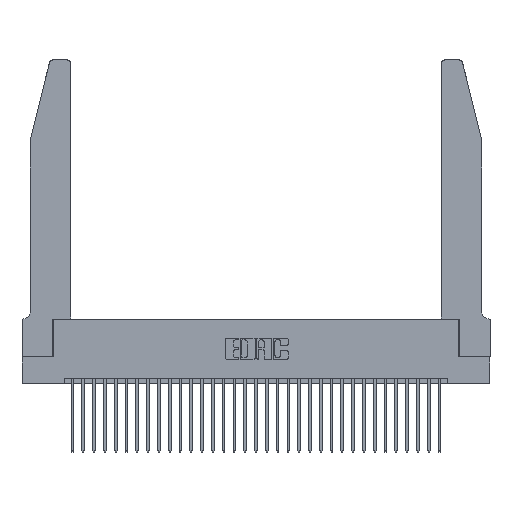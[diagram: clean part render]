
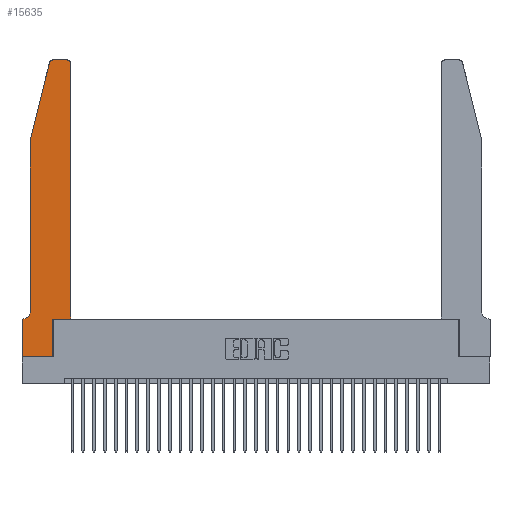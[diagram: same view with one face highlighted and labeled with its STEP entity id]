
A CAD part, top view. The second image highlights one B-rep face of the part: STEP entity #15635.
In plain terms, the highlighted planar face has unit normal (0, 0, 1).
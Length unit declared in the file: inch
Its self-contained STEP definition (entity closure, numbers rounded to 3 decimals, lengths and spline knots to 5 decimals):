
#44 = ORIENTED_EDGE ( 'NONE', *, *, #20738, .T. ) ;
#1139 = EDGE_CURVE ( 'NONE', #29773, #28046, #31477, .T. ) ;
#1188 = DIRECTION ( 'NONE',  ( 1., 0., 0. ) ) ;
#1494 = DIRECTION ( 'NONE',  ( -1., 0., 0. ) ) ;
#2541 = LINE ( 'NONE', #8914, #22232 ) ;
#2862 = ORIENTED_EDGE ( 'NONE', *, *, #24527, .T. ) ;
#3100 = AXIS2_PLACEMENT_3D ( 'NONE', #10917, #31231, #28547 ) ;
#3407 = DIRECTION ( 'NONE',  ( 0., 1., 0. ) ) ;
#3511 = LINE ( 'NONE', #30862, #12816 ) ;
#3593 = ORIENTED_EDGE ( 'NONE', *, *, #30629, .T. ) ;
#3734 = VERTEX_POINT ( 'NONE', #26881 ) ;
#4001 = CARTESIAN_POINT ( 'NONE',  ( 0.2865, 0.35, 0.37 ) ) ;
#4684 = ORIENTED_EDGE ( 'NONE', *, *, #8996, .T. ) ;
#5107 = DIRECTION ( 'NONE',  ( 0., 0., -1. ) ) ;
#5984 = EDGE_CURVE ( 'NONE', #23212, #20855, #3511, .T. ) ;
#6069 = VERTEX_POINT ( 'NONE', #24100 ) ;
#6138 = CARTESIAN_POINT ( 'NONE',  ( 0.284, 2.75, 0.37 ) ) ;
#7278 = CARTESIAN_POINT ( 'NONE',  ( 0.0055, 0.42, 0.37 ) ) ;
#7565 = ORIENTED_EDGE ( 'NONE', *, *, #8165, .T. ) ;
#7807 = LINE ( 'NONE', #10770, #21006 ) ;
#7974 = ORIENTED_EDGE ( 'NONE', *, *, #15276, .T. ) ;
#7991 = EDGE_LOOP ( 'NONE', ( #7565, #32220, #29162, #4684, #2862, #28185, #7974, #3593, #24449, #31162, #17124, #44 ) ) ;
#8165 = EDGE_CURVE ( 'NONE', #8243, #15471, #18861, .T. ) ;
#8214 = VECTOR ( 'NONE', #21983, 39.37008 ) ;
#8243 = VERTEX_POINT ( 'NONE', #17296 ) ;
#8914 = CARTESIAN_POINT ( 'NONE',  ( 0.4505, 0.35, 0.37 ) ) ;
#8996 = EDGE_CURVE ( 'NONE', #20855, #14563, #14659, .T. ) ;
#9377 = VECTOR ( 'NONE', #3407, 39.37008 ) ;
#10770 = CARTESIAN_POINT ( 'NONE',  ( 0., 0., 0.37 ) ) ;
#10917 = CARTESIAN_POINT ( 'NONE',  ( 0.4205, 2.72, 0.37 ) ) ;
#11290 = DIRECTION ( 'NONE',  ( 1., 0., 0. ) ) ;
#11753 = VERTEX_POINT ( 'NONE', #12841 ) ;
#12213 = EDGE_CURVE ( 'NONE', #29085, #6069, #20867, .T. ) ;
#12527 = VECTOR ( 'NONE', #17691, 39.37008 ) ;
#12816 = VECTOR ( 'NONE', #25686, 39.37008 ) ;
#12841 = CARTESIAN_POINT ( 'NONE',  ( 0., 0., 0.37 ) ) ;
#13200 = CARTESIAN_POINT ( 'NONE',  ( 0.4505, 2.72, 0.37 ) ) ;
#13548 = DIRECTION ( 'NONE',  ( 0., 0., 1. ) ) ;
#13605 = AXIS2_PLACEMENT_3D ( 'NONE', #7278, #5107, #15448 ) ;
#13682 = DIRECTION ( 'NONE',  ( -1., 0., 0. ) ) ;
#13918 = CIRCLE ( 'NONE', #13605, 0.07 ) ;
#14563 = VERTEX_POINT ( 'NONE', #17896 ) ;
#14659 = LINE ( 'NONE', #27059, #26262 ) ;
#15276 = EDGE_CURVE ( 'NONE', #6069, #11753, #7807, .T. ) ;
#15448 = DIRECTION ( 'NONE',  ( -1., 0., 0. ) ) ;
#15471 = VERTEX_POINT ( 'NONE', #6138 ) ;
#15635 = ADVANCED_FACE ( 'NONE', ( #29424 ), #26188, .T. ) ;
#15729 = EDGE_CURVE ( 'NONE', #28046, #3734, #2541, .T. ) ;
#16372 = CARTESIAN_POINT ( 'NONE',  ( 0.0755, 0.35, 0.37 ) ) ;
#16467 = VECTOR ( 'NONE', #1494, 39.37008 ) ;
#16550 = CARTESIAN_POINT ( 'NONE',  ( 0.0055, 0.35, 0.37 ) ) ;
#16721 = AXIS2_PLACEMENT_3D ( 'NONE', #33086, #18148, #20621 ) ;
#16952 = CARTESIAN_POINT ( 'NONE',  ( 0.2865, 0., 0.37 ) ) ;
#17124 = ORIENTED_EDGE ( 'NONE', *, *, #25946, .T. ) ;
#17213 = CARTESIAN_POINT ( 'NONE',  ( 0.0755, 2., 0.37 ) ) ;
#17296 = CARTESIAN_POINT ( 'NONE',  ( 0.4205, 2.75, 0.37 ) ) ;
#17691 = DIRECTION ( 'NONE',  ( 1., 0., 0. ) ) ;
#17896 = CARTESIAN_POINT ( 'NONE',  ( 0.0755, 0.42, 0.37 ) ) ;
#18148 = DIRECTION ( 'NONE',  ( 0., 0., 1. ) ) ;
#18810 = CARTESIAN_POINT ( 'NONE',  ( 0.4505, 0.35, 0.37 ) ) ;
#18861 = LINE ( 'NONE', #24466, #16467 ) ;
#19808 = CIRCLE ( 'NONE', #16721, 0.03 ) ;
#20621 = DIRECTION ( 'NONE',  ( 1., 0., 0. ) ) ;
#20738 = EDGE_CURVE ( 'NONE', #22619, #8243, #25141, .T. ) ;
#20855 = VERTEX_POINT ( 'NONE', #17213 ) ;
#20867 = LINE ( 'NONE', #16372, #26501 ) ;
#21006 = VECTOR ( 'NONE', #28832, 39.37008 ) ;
#21983 = DIRECTION ( 'NONE',  ( 0., 1., 0. ) ) ;
#22232 = VECTOR ( 'NONE', #1188, 39.37008 ) ;
#22619 = VERTEX_POINT ( 'NONE', #13200 ) ;
#23212 = VERTEX_POINT ( 'NONE', #26747 ) ;
#24100 = CARTESIAN_POINT ( 'NONE',  ( 0., 0.35, 0.37 ) ) ;
#24163 = LINE ( 'NONE', #33039, #12527 ) ;
#24240 = LINE ( 'NONE', #18810, #9377 ) ;
#24449 = ORIENTED_EDGE ( 'NONE', *, *, #1139, .T. ) ;
#24466 = CARTESIAN_POINT ( 'NONE',  ( 0.2605, 2.75, 0.37 ) ) ;
#24527 = EDGE_CURVE ( 'NONE', #14563, #29085, #13918, .T. ) ;
#25141 = CIRCLE ( 'NONE', #3100, 0.03 ) ;
#25686 = DIRECTION ( 'NONE',  ( -0.239, -0.971, 0. ) ) ;
#25946 = EDGE_CURVE ( 'NONE', #3734, #22619, #24240, .T. ) ;
#26188 = PLANE ( 'NONE',  #28200 ) ;
#26262 = VECTOR ( 'NONE', #26473, 39.37008 ) ;
#26473 = DIRECTION ( 'NONE',  ( 0., -1., 0. ) ) ;
#26501 = VECTOR ( 'NONE', #13682, 39.37008 ) ;
#26747 = CARTESIAN_POINT ( 'NONE',  ( 0.25487, 2.72718, 0.37 ) ) ;
#26881 = CARTESIAN_POINT ( 'NONE',  ( 0.4505, 0.35, 0.37 ) ) ;
#27059 = CARTESIAN_POINT ( 'NONE',  ( 0.0755, 2., 0.37 ) ) ;
#28046 = VERTEX_POINT ( 'NONE', #29930 ) ;
#28185 = ORIENTED_EDGE ( 'NONE', *, *, #12213, .T. ) ;
#28200 = AXIS2_PLACEMENT_3D ( 'NONE', #28672, #13548, #11290 ) ;
#28547 = DIRECTION ( 'NONE',  ( 1., 0., 0. ) ) ;
#28672 = CARTESIAN_POINT ( 'NONE',  ( 0., 0.35, 0.37 ) ) ;
#28832 = DIRECTION ( 'NONE',  ( 0., -1., 0. ) ) ;
#29085 = VERTEX_POINT ( 'NONE', #16550 ) ;
#29162 = ORIENTED_EDGE ( 'NONE', *, *, #5984, .T. ) ;
#29424 = FACE_OUTER_BOUND ( 'NONE', #7991, .T. ) ;
#29773 = VERTEX_POINT ( 'NONE', #16952 ) ;
#29930 = CARTESIAN_POINT ( 'NONE',  ( 0.2865, 0.35, 0.37 ) ) ;
#30099 = EDGE_CURVE ( 'NONE', #15471, #23212, #19808, .T. ) ;
#30629 = EDGE_CURVE ( 'NONE', #11753, #29773, #24163, .T. ) ;
#30862 = CARTESIAN_POINT ( 'NONE',  ( 0.0755, 2., 0.37 ) ) ;
#31162 = ORIENTED_EDGE ( 'NONE', *, *, #15729, .T. ) ;
#31231 = DIRECTION ( 'NONE',  ( 0., 0., 1. ) ) ;
#31477 = LINE ( 'NONE', #4001, #8214 ) ;
#32220 = ORIENTED_EDGE ( 'NONE', *, *, #30099, .T. ) ;
#33039 = CARTESIAN_POINT ( 'NONE',  ( 0., 0., 0.37 ) ) ;
#33086 = CARTESIAN_POINT ( 'NONE',  ( 0.284, 2.72, 0.37 ) ) ;
